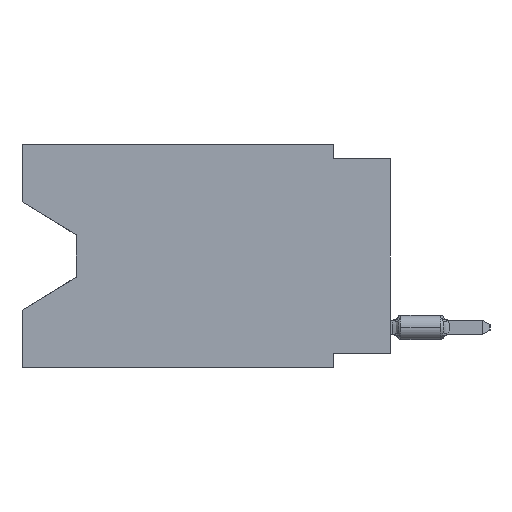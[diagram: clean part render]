
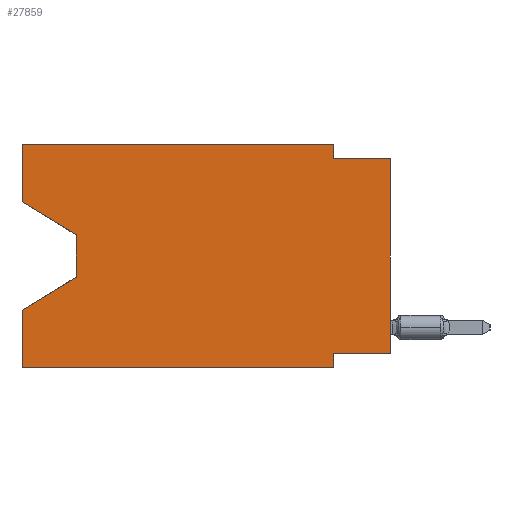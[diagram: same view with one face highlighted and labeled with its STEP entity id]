
A CAD part, left-side view. The second image highlights one B-rep face of the part: STEP entity #27859.
In plain terms, the highlighted planar face has unit normal (-1, 0, 0).
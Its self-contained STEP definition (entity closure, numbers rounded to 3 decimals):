
#384 = ORIENTED_EDGE ( 'NONE', *, *, #10287, .T. ) ;
#2899 = DIRECTION ( 'NONE',  ( 0., 0., -1. ) ) ;
#3224 = LINE ( 'NONE', #33065, #20254 ) ;
#4799 = CARTESIAN_POINT ( 'NONE',  ( 0., 16.383, 0. ) ) ;
#4975 = EDGE_CURVE ( 'NONE', #40465, #54520, #12789, .T. ) ;
#5258 = CARTESIAN_POINT ( 'NONE',  ( 0., 16.383, -7.36 ) ) ;
#6085 = CARTESIAN_POINT ( 'NONE',  ( 0., 13.97, -4.013 ) ) ;
#6617 = CARTESIAN_POINT ( 'NONE',  ( 0., 2.54, -9.271 ) ) ;
#6657 = VECTOR ( 'NONE', #39557, 1000. ) ;
#8298 = DIRECTION ( 'NONE',  ( 0., 0., 1. ) ) ;
#8321 = VECTOR ( 'NONE', #48052, 1000. ) ;
#8605 = VECTOR ( 'NONE', #27347, 1000. ) ;
#8788 = CARTESIAN_POINT ( 'NONE',  ( 0., 16.383, 0. ) ) ;
#9399 = VECTOR ( 'NONE', #27878, 1000. ) ;
#10287 = EDGE_CURVE ( 'NONE', #61229, #14112, #24350, .T. ) ;
#10290 = VERTEX_POINT ( 'NONE', #28631 ) ;
#11138 = ORIENTED_EDGE ( 'NONE', *, *, #50855, .F. ) ;
#11625 = ORIENTED_EDGE ( 'NONE', *, *, #50927, .F. ) ;
#12185 = ORIENTED_EDGE ( 'NONE', *, *, #58883, .T. ) ;
#12789 = LINE ( 'NONE', #23595, #9399 ) ;
#13256 = EDGE_CURVE ( 'NONE', #53798, #49851, #62463, .T. ) ;
#14112 = VERTEX_POINT ( 'NONE', #56725 ) ;
#15046 = CARTESIAN_POINT ( 'NONE',  ( 0., 2.54, -0.635 ) ) ;
#16771 = VECTOR ( 'NONE', #29099, 1000. ) ;
#17183 = CARTESIAN_POINT ( 'NONE',  ( 0., 13.97, -5.893 ) ) ;
#18604 = DIRECTION ( 'NONE',  ( 0., -0.855, -0.519 ) ) ;
#20254 = VECTOR ( 'NONE', #18604, 1000. ) ;
#21038 = ORIENTED_EDGE ( 'NONE', *, *, #64114, .T. ) ;
#21129 = ORIENTED_EDGE ( 'NONE', *, *, #13256, .F. ) ;
#22099 = LINE ( 'NONE', #17183, #8605 ) ;
#22251 = DIRECTION ( 'NONE',  ( 1., 0., 0. ) ) ;
#23395 = DIRECTION ( 'NONE',  ( 0., -1., 0. ) ) ;
#23557 = LINE ( 'NONE', #27840, #48372 ) ;
#23595 = CARTESIAN_POINT ( 'NONE',  ( 0., 0., -0.635 ) ) ;
#23690 = CARTESIAN_POINT ( 'NONE',  ( 0., 0., -9.271 ) ) ;
#23772 = VERTEX_POINT ( 'NONE', #23690 ) ;
#24350 = LINE ( 'NONE', #39752, #50677 ) ;
#24793 = VERTEX_POINT ( 'NONE', #41988 ) ;
#24876 = LINE ( 'NONE', #6085, #30132 ) ;
#25131 = EDGE_LOOP ( 'NONE', ( #29926, #59923, #21038, #11138, #384, #11625, #51912, #12185, #61495, #32456, #21129, #62941 ) ) ;
#27077 = VECTOR ( 'NONE', #8298, 1000. ) ;
#27347 = DIRECTION ( 'NONE',  ( 0., 0.855, -0.519 ) ) ;
#27840 = CARTESIAN_POINT ( 'NONE',  ( 0., 2.54, -9.906 ) ) ;
#27859 = ADVANCED_FACE ( 'NONE', ( #46855 ), #32740, .F. ) ;
#27878 = DIRECTION ( 'NONE',  ( 0., -1., 0. ) ) ;
#28631 = CARTESIAN_POINT ( 'NONE',  ( 0., 13.97, -5.893 ) ) ;
#29099 = DIRECTION ( 'NONE',  ( 0., 1., 0. ) ) ;
#29811 = DIRECTION ( 'NONE',  ( 0., 0., -1. ) ) ;
#29926 = ORIENTED_EDGE ( 'NONE', *, *, #53792, .T. ) ;
#30132 = VECTOR ( 'NONE', #29811, 1000. ) ;
#32456 = ORIENTED_EDGE ( 'NONE', *, *, #58364, .F. ) ;
#32740 = PLANE ( 'NONE',  #57704 ) ;
#32930 = CARTESIAN_POINT ( 'NONE',  ( 0., 16.383, 0. ) ) ;
#33065 = CARTESIAN_POINT ( 'NONE',  ( 0., 16.383, -2.546 ) ) ;
#33694 = LINE ( 'NONE', #44503, #16771 ) ;
#35267 = LINE ( 'NONE', #4799, #6657 ) ;
#36707 = LINE ( 'NONE', #50832, #52550 ) ;
#37112 = EDGE_CURVE ( 'NONE', #50401, #10290, #24876, .T. ) ;
#38229 = EDGE_CURVE ( 'NONE', #24793, #53798, #35267, .T. ) ;
#39429 = LINE ( 'NONE', #58145, #27077 ) ;
#39557 = DIRECTION ( 'NONE',  ( 0., 0., 1. ) ) ;
#39752 = CARTESIAN_POINT ( 'NONE',  ( 0., 16.383, -9.906 ) ) ;
#40465 = VERTEX_POINT ( 'NONE', #15046 ) ;
#41988 = CARTESIAN_POINT ( 'NONE',  ( 0., 16.383, -2.546 ) ) ;
#44503 = CARTESIAN_POINT ( 'NONE',  ( 0., 0., -9.271 ) ) ;
#44558 = CARTESIAN_POINT ( 'NONE',  ( 0., 16.383, -9.906 ) ) ;
#46855 = FACE_OUTER_BOUND ( 'NONE', #25131, .T. ) ;
#47534 = DIRECTION ( 'NONE',  ( 0., 0., -1. ) ) ;
#48052 = DIRECTION ( 'NONE',  ( 0., 0., -1. ) ) ;
#48372 = VECTOR ( 'NONE', #47534, 1000. ) ;
#49851 = VERTEX_POINT ( 'NONE', #54699 ) ;
#50401 = VERTEX_POINT ( 'NONE', #51234 ) ;
#50677 = VECTOR ( 'NONE', #64364, 1000. ) ;
#50832 = CARTESIAN_POINT ( 'NONE',  ( 0., 16.383, 0. ) ) ;
#50855 = EDGE_CURVE ( 'NONE', #61229, #62776, #36707, .T. ) ;
#50927 = EDGE_CURVE ( 'NONE', #54744, #14112, #23557, .T. ) ;
#51234 = CARTESIAN_POINT ( 'NONE',  ( 0., 13.97, -4.013 ) ) ;
#51809 = DIRECTION ( 'NONE',  ( 0., 0., 1. ) ) ;
#51912 = ORIENTED_EDGE ( 'NONE', *, *, #60045, .F. ) ;
#51959 = CARTESIAN_POINT ( 'NONE',  ( 0., 0., -0.635 ) ) ;
#52550 = VECTOR ( 'NONE', #51809, 1000. ) ;
#52972 = CARTESIAN_POINT ( 'NONE',  ( 0., 2.54, 0. ) ) ;
#53792 = EDGE_CURVE ( 'NONE', #24793, #50401, #3224, .T. ) ;
#53798 = VERTEX_POINT ( 'NONE', #8788 ) ;
#54520 = VERTEX_POINT ( 'NONE', #51959 ) ;
#54699 = CARTESIAN_POINT ( 'NONE',  ( 0., 2.54, 0. ) ) ;
#54744 = VERTEX_POINT ( 'NONE', #6617 ) ;
#56725 = CARTESIAN_POINT ( 'NONE',  ( 0., 2.54, -9.906 ) ) ;
#57023 = CARTESIAN_POINT ( 'NONE',  ( 0., 16.383, 0. ) ) ;
#57258 = LINE ( 'NONE', #52972, #8321 ) ;
#57704 = AXIS2_PLACEMENT_3D ( 'NONE', #57023, #22251, #2899 ) ;
#58145 = CARTESIAN_POINT ( 'NONE',  ( 0., 0., 0. ) ) ;
#58364 = EDGE_CURVE ( 'NONE', #49851, #40465, #57258, .T. ) ;
#58883 = EDGE_CURVE ( 'NONE', #23772, #54520, #39429, .T. ) ;
#59923 = ORIENTED_EDGE ( 'NONE', *, *, #37112, .T. ) ;
#60045 = EDGE_CURVE ( 'NONE', #23772, #54744, #33694, .T. ) ;
#61229 = VERTEX_POINT ( 'NONE', #44558 ) ;
#61495 = ORIENTED_EDGE ( 'NONE', *, *, #4975, .F. ) ;
#61522 = VECTOR ( 'NONE', #23395, 1000. ) ;
#62463 = LINE ( 'NONE', #32930, #61522 ) ;
#62776 = VERTEX_POINT ( 'NONE', #5258 ) ;
#62941 = ORIENTED_EDGE ( 'NONE', *, *, #38229, .F. ) ;
#64114 = EDGE_CURVE ( 'NONE', #10290, #62776, #22099, .T. ) ;
#64364 = DIRECTION ( 'NONE',  ( 0., -1., 0. ) ) ;
